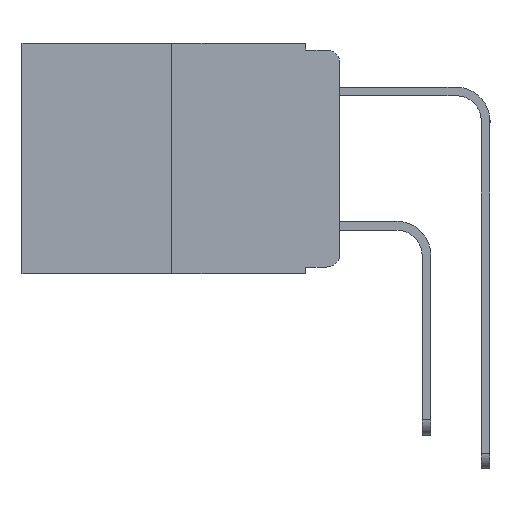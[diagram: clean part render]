
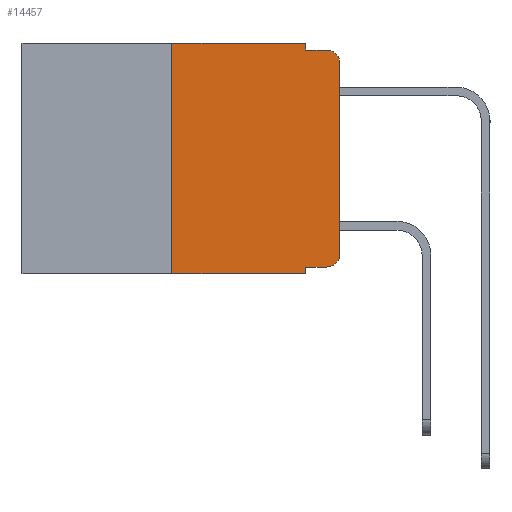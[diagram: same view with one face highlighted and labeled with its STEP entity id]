
A CAD part, left-side view. The second image highlights one B-rep face of the part: STEP entity #14457.
In plain terms, the highlighted planar face has unit normal (-1, 0, 0).
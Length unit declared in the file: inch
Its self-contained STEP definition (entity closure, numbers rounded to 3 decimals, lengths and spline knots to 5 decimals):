
#244 = LINE ( 'NONE', #8348, #7799 ) ;
#602 = VERTEX_POINT ( 'NONE', #7863 ) ;
#972 = CARTESIAN_POINT ( 'NONE',  ( 0., 0.473, 0. ) ) ;
#1218 = AXIS2_PLACEMENT_3D ( 'NONE', #16987, #8414, #18430 ) ;
#1371 = CARTESIAN_POINT ( 'NONE',  ( 0., 0.25, -0.343 ) ) ;
#1890 = DIRECTION ( 'NONE',  ( 0., 0., 1. ) ) ;
#2299 = VECTOR ( 'NONE', #8225, 39.37008 ) ;
#2348 = DIRECTION ( 'NONE',  ( -1., 0., 0. ) ) ;
#2491 = CARTESIAN_POINT ( 'NONE',  ( 0., 0.051, 0. ) ) ;
#3285 = CARTESIAN_POINT ( 'NONE',  ( 0., 0., -0.03 ) ) ;
#3529 = VERTEX_POINT ( 'NONE', #12710 ) ;
#3546 = DIRECTION ( 'NONE',  ( 1., 0., 0. ) ) ;
#3796 = LINE ( 'NONE', #15052, #16755 ) ;
#3895 = CARTESIAN_POINT ( 'NONE',  ( 0., 0.25, 0. ) ) ;
#3961 = DIRECTION ( 'NONE',  ( 0., 0., 1. ) ) ;
#4178 = CARTESIAN_POINT ( 'NONE',  ( 0., 0.473, -0.343 ) ) ;
#4240 = VERTEX_POINT ( 'NONE', #11060 ) ;
#4486 = VECTOR ( 'NONE', #12701, 39.37008 ) ;
#4893 = VERTEX_POINT ( 'NONE', #3285 ) ;
#4897 = VECTOR ( 'NONE', #5598, 39.37008 ) ;
#5308 = LINE ( 'NONE', #3895, #8673 ) ;
#5598 = DIRECTION ( 'NONE',  ( 0., -1., 0. ) ) ;
#5778 = CIRCLE ( 'NONE', #15222, 0.02 ) ;
#6248 = VECTOR ( 'NONE', #1890, 39.37008 ) ;
#6505 = DIRECTION ( 'NONE',  ( 0., -1., 0. ) ) ;
#6545 = CARTESIAN_POINT ( 'NONE',  ( 0., 0.051, -0.333 ) ) ;
#6573 = VERTEX_POINT ( 'NONE', #1371 ) ;
#7313 = EDGE_LOOP ( 'NONE', ( #16819, #17038, #17942, #13537, #12805, #11425, #11407, #15957, #12595, #12458 ) ) ;
#7799 = VECTOR ( 'NONE', #11212, 39.37008 ) ;
#7863 = CARTESIAN_POINT ( 'NONE',  ( 0., 0.02, -0.01 ) ) ;
#8225 = DIRECTION ( 'NONE',  ( 0., 0., -1. ) ) ;
#8237 = VECTOR ( 'NONE', #16864, 39.37008 ) ;
#8348 = CARTESIAN_POINT ( 'NONE',  ( 0., 0.051, -0.333 ) ) ;
#8414 = DIRECTION ( 'NONE',  ( -1., 0., 0. ) ) ;
#8498 = EDGE_CURVE ( 'NONE', #17665, #3529, #11164, .T. ) ;
#8673 = VECTOR ( 'NONE', #3961, 39.37008 ) ;
#8820 = EDGE_CURVE ( 'NONE', #6573, #4240, #16766, .T. ) ;
#9123 = EDGE_CURVE ( 'NONE', #18597, #4893, #10472, .T. ) ;
#9127 = LINE ( 'NONE', #18241, #2299 ) ;
#9149 = EDGE_CURVE ( 'NONE', #4893, #602, #5778, .T. ) ;
#9150 = EDGE_CURVE ( 'NONE', #11523, #602, #3796, .T. ) ;
#9171 = EDGE_CURVE ( 'NONE', #3529, #11523, #9127, .T. ) ;
#9176 = EDGE_CURVE ( 'NONE', #6573, #17665, #5308, .T. ) ;
#9201 = EDGE_CURVE ( 'NONE', #14521, #4240, #12508, .T. ) ;
#9222 = EDGE_CURVE ( 'NONE', #14521, #13024, #244, .T. ) ;
#9229 = EDGE_CURVE ( 'NONE', #13024, #18597, #15410, .T. ) ;
#10431 = CARTESIAN_POINT ( 'NONE',  ( 0., 0.051, -0.01 ) ) ;
#10472 = LINE ( 'NONE', #10653, #6248 ) ;
#10653 = CARTESIAN_POINT ( 'NONE',  ( 0., 0., 0. ) ) ;
#10690 = CARTESIAN_POINT ( 'NONE',  ( 0., 0.473, 0. ) ) ;
#11012 = CARTESIAN_POINT ( 'NONE',  ( 0., 0.02, -0.03 ) ) ;
#11060 = CARTESIAN_POINT ( 'NONE',  ( 0., 0.051, -0.343 ) ) ;
#11164 = LINE ( 'NONE', #972, #4486 ) ;
#11212 = DIRECTION ( 'NONE',  ( 0., -1., 0. ) ) ;
#11407 = ORIENTED_EDGE ( 'NONE', *, *, #8820, .T. ) ;
#11425 = ORIENTED_EDGE ( 'NONE', *, *, #9176, .F. ) ;
#11523 = VERTEX_POINT ( 'NONE', #10431 ) ;
#12189 = CARTESIAN_POINT ( 'NONE',  ( 0., 0., -0.313 ) ) ;
#12458 = ORIENTED_EDGE ( 'NONE', *, *, #9229, .T. ) ;
#12496 = DIRECTION ( 'NONE',  ( 0., 0., -1. ) ) ;
#12508 = LINE ( 'NONE', #2491, #8237 ) ;
#12595 = ORIENTED_EDGE ( 'NONE', *, *, #9222, .T. ) ;
#12701 = DIRECTION ( 'NONE',  ( 0., -1., 0. ) ) ;
#12710 = CARTESIAN_POINT ( 'NONE',  ( 0., 0.051, 0. ) ) ;
#12805 = ORIENTED_EDGE ( 'NONE', *, *, #8498, .F. ) ;
#13024 = VERTEX_POINT ( 'NONE', #13608 ) ;
#13537 = ORIENTED_EDGE ( 'NONE', *, *, #9171, .F. ) ;
#13608 = CARTESIAN_POINT ( 'NONE',  ( 0., 0.02, -0.333 ) ) ;
#13612 = DIRECTION ( 'NONE',  ( 0., 0., -1. ) ) ;
#14457 = ADVANCED_FACE ( 'NONE', ( #17260 ), #14980, .F. ) ;
#14521 = VERTEX_POINT ( 'NONE', #6545 ) ;
#14980 = PLANE ( 'NONE',  #18056 ) ;
#15052 = CARTESIAN_POINT ( 'NONE',  ( 0., 0.051, -0.01 ) ) ;
#15222 = AXIS2_PLACEMENT_3D ( 'NONE', #11012, #2348, #12496 ) ;
#15410 = CIRCLE ( 'NONE', #1218, 0.02 ) ;
#15957 = ORIENTED_EDGE ( 'NONE', *, *, #9201, .F. ) ;
#16755 = VECTOR ( 'NONE', #6505, 39.37008 ) ;
#16766 = LINE ( 'NONE', #4178, #4897 ) ;
#16819 = ORIENTED_EDGE ( 'NONE', *, *, #9123, .T. ) ;
#16864 = DIRECTION ( 'NONE',  ( 0., 0., -1. ) ) ;
#16977 = CARTESIAN_POINT ( 'NONE',  ( 0., 0.25, 0. ) ) ;
#16987 = CARTESIAN_POINT ( 'NONE',  ( 0., 0.02, -0.313 ) ) ;
#17038 = ORIENTED_EDGE ( 'NONE', *, *, #9149, .T. ) ;
#17260 = FACE_OUTER_BOUND ( 'NONE', #7313, .T. ) ;
#17665 = VERTEX_POINT ( 'NONE', #16977 ) ;
#17942 = ORIENTED_EDGE ( 'NONE', *, *, #9150, .F. ) ;
#18056 = AXIS2_PLACEMENT_3D ( 'NONE', #10690, #3546, #13612 ) ;
#18241 = CARTESIAN_POINT ( 'NONE',  ( 0., 0.051, 0. ) ) ;
#18430 = DIRECTION ( 'NONE',  ( 0., 0., -1. ) ) ;
#18597 = VERTEX_POINT ( 'NONE', #12189 ) ;
